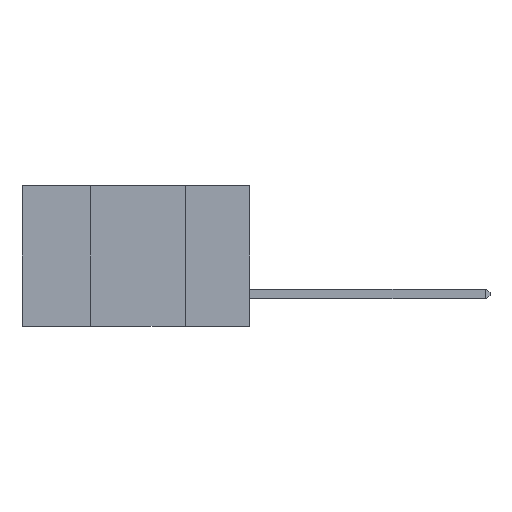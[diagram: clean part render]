
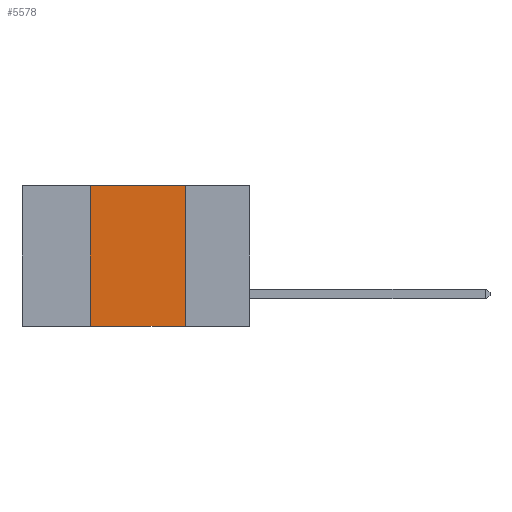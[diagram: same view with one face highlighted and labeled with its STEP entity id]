
A CAD part, left-side view. The second image highlights one B-rep face of the part: STEP entity #5578.
In plain terms, the highlighted planar face has unit normal (-1, 0, 0).
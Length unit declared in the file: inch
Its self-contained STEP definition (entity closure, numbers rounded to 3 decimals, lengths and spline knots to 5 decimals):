
#696 = LINE ( 'NONE', #5821, #7823 ) ;
#899 = DIRECTION ( 'NONE',  ( 0., -1., 0. ) ) ;
#982 = CARTESIAN_POINT ( 'NONE',  ( 0., 0.6, -0.37 ) ) ;
#1434 = EDGE_CURVE ( 'NONE', #3528, #4818, #696, .T. ) ;
#1504 = VERTEX_POINT ( 'NONE', #4567 ) ;
#1662 = LINE ( 'NONE', #982, #8721 ) ;
#2443 = VECTOR ( 'NONE', #8528, 39.37008 ) ;
#2587 = LINE ( 'NONE', #5630, #5888 ) ;
#3528 = VERTEX_POINT ( 'NONE', #3543 ) ;
#3543 = CARTESIAN_POINT ( 'NONE',  ( 0., 0.17, 0. ) ) ;
#3740 = FACE_OUTER_BOUND ( 'NONE', #4504, .T. ) ;
#3882 = EDGE_CURVE ( 'NONE', #7537, #1504, #2587, .T. ) ;
#4009 = CARTESIAN_POINT ( 'NONE',  ( 0., 0.17, -0.37 ) ) ;
#4381 = EDGE_CURVE ( 'NONE', #7537, #4818, #1662, .T. ) ;
#4383 = LINE ( 'NONE', #6099, #2443 ) ;
#4504 = EDGE_LOOP ( 'NONE', ( #7055, #6652, #6143, #5588 ) ) ;
#4567 = CARTESIAN_POINT ( 'NONE',  ( 0., 0.42, 0. ) ) ;
#4634 = DIRECTION ( 'NONE',  ( 0., 0., 1. ) ) ;
#4818 = VERTEX_POINT ( 'NONE', #4009 ) ;
#4902 = DIRECTION ( 'NONE',  ( 0., 0., -1. ) ) ;
#4919 = DIRECTION ( 'NONE',  ( 1., 0., 0. ) ) ;
#4945 = PLANE ( 'NONE',  #5025 ) ;
#4951 = CARTESIAN_POINT ( 'NONE',  ( 0., 0.6, 0. ) ) ;
#5025 = AXIS2_PLACEMENT_3D ( 'NONE', #4951, #4919, #4902 ) ;
#5578 = ADVANCED_FACE ( 'NONE', ( #3740 ), #4945, .F. ) ;
#5588 = ORIENTED_EDGE ( 'NONE', *, *, #4381, .T. ) ;
#5630 = CARTESIAN_POINT ( 'NONE',  ( 0., 0.42, 0. ) ) ;
#5750 = CARTESIAN_POINT ( 'NONE',  ( 0., 0.42, -0.37 ) ) ;
#5821 = CARTESIAN_POINT ( 'NONE',  ( 0., 0.17, 0. ) ) ;
#5888 = VECTOR ( 'NONE', #4634, 39.37008 ) ;
#6099 = CARTESIAN_POINT ( 'NONE',  ( 0., 0.6, 0. ) ) ;
#6143 = ORIENTED_EDGE ( 'NONE', *, *, #3882, .F. ) ;
#6652 = ORIENTED_EDGE ( 'NONE', *, *, #8499, .F. ) ;
#7016 = DIRECTION ( 'NONE',  ( 0., 0., -1. ) ) ;
#7055 = ORIENTED_EDGE ( 'NONE', *, *, #1434, .F. ) ;
#7537 = VERTEX_POINT ( 'NONE', #5750 ) ;
#7823 = VECTOR ( 'NONE', #7016, 39.37008 ) ;
#8499 = EDGE_CURVE ( 'NONE', #1504, #3528, #4383, .T. ) ;
#8528 = DIRECTION ( 'NONE',  ( 0., -1., 0. ) ) ;
#8721 = VECTOR ( 'NONE', #899, 39.37008 ) ;
